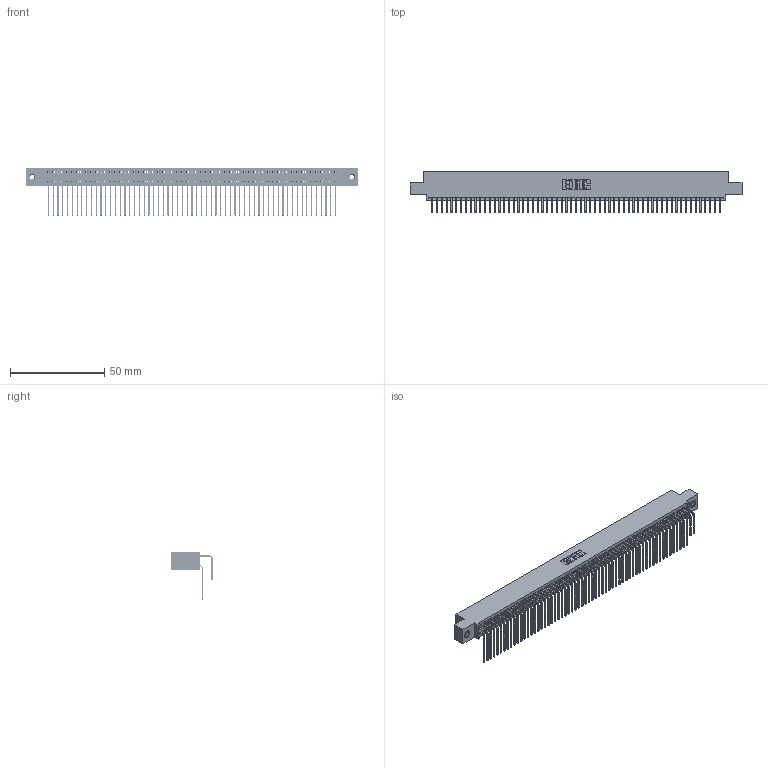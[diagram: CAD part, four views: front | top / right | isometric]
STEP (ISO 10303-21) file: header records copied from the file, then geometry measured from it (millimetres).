
FILE_DESCRIPTION (( 'STEP AP203' ), '1' );
FILE_NAME ('845-122-558-508.STEP', '2018-11-21T14:12:34', ( '' ), ( '' ), 'SwSTEP 2.0', 'SolidWorks 2016', '' );
FILE_SCHEMA (( 'CONFIG_CONTROL_DESIGN' ));
Length unit declared in the file: inch
Products named in the file (5): 845 Part_0.110 Offset - 0.156 Dia-TI; 345-292-001_558 559 Tail - 1; 345-292-001_558 Tail - 2; 345-250-001_345-250-003-102; 845-122-558-508
Assembly tree (125 placements, depth 2):
  845-122-558-508
    845 Part_0.110 Offset - 0.156 Dia-TI
    345-292-001_558 559 Tail - 1  x61
    345-292-001_558 Tail - 2  x61
    345-250-001_345-250-003-102  x2
Bounding box: 176.15 x 21.83 x 25.53 mm (x, y, z)
Volume: 17009.8 mm3; surface area: 30254.5 mm2
Topology: 64 solids, 125 shells, 6534 faces, 19399 edges, 12701 vertices
Faces by surface type: plane 4386, cylinder 2132, cone 12, torus 4
Entity records: 48274 total; most frequent: CARTESIAN_POINT 8102, ORIENTED_EDGE 7978, DIRECTION 7119, EDGE_CURVE 3989, VECTOR 3553, LINE 3553, VERTEX_POINT 2652, AXIS2_PLACEMENT_3D 1783
